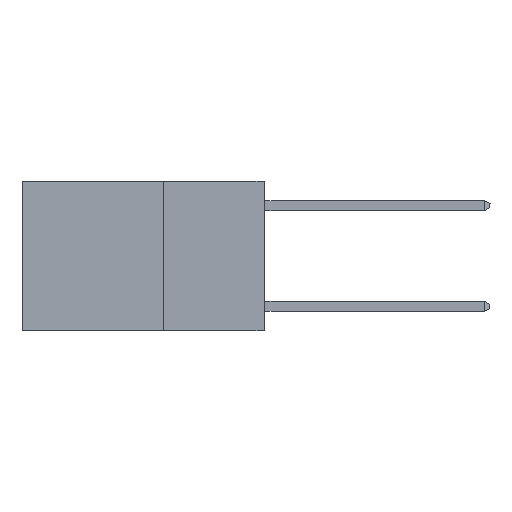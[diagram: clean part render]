
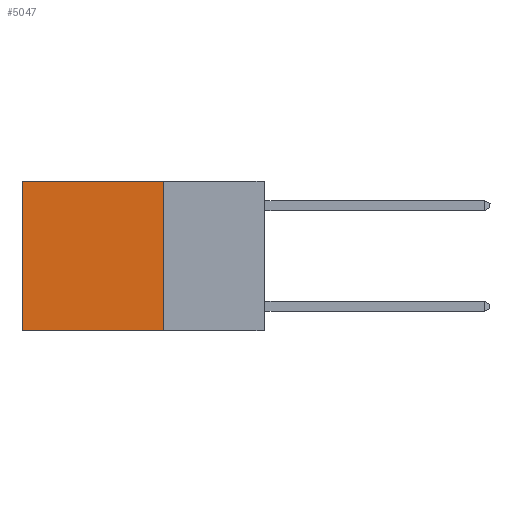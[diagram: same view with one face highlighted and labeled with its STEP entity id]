
A CAD part, left-side view. The second image highlights one B-rep face of the part: STEP entity #5047.
In plain terms, the highlighted planar face has unit normal (-1, 0, 0).
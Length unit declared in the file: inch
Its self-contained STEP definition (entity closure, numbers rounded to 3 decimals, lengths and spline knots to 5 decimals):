
#26 = DIRECTION ( 'NONE',  ( 0., 1., 0. ) ) ;
#517 = ORIENTED_EDGE ( 'NONE', *, *, #11591, .F. ) ;
#557 = ORIENTED_EDGE ( 'NONE', *, *, #10270, .T. ) ;
#686 = VECTOR ( 'NONE', #26, 39.37008 ) ;
#772 = ORIENTED_EDGE ( 'NONE', *, *, #4914, .F. ) ;
#889 = ORIENTED_EDGE ( 'NONE', *, *, #3228, .T. ) ;
#1190 = VERTEX_POINT ( 'NONE', #11742 ) ;
#1221 = VERTEX_POINT ( 'NONE', #10866 ) ;
#1731 = DIRECTION ( 'NONE',  ( 0., 0., -1. ) ) ;
#3228 = EDGE_CURVE ( 'NONE', #4956, #6445, #5543, .T. ) ;
#3230 = AXIS2_PLACEMENT_3D ( 'NONE', #3625, #7593, #1731 ) ;
#3414 = CARTESIAN_POINT ( 'NONE',  ( 0.2625, 0.25, 0. ) ) ;
#3625 = CARTESIAN_POINT ( 'NONE',  ( 0.2625, 0.25, 0. ) ) ;
#4360 = CARTESIAN_POINT ( 'NONE',  ( 0.2625, 0.25, 0. ) ) ;
#4914 = EDGE_CURVE ( 'NONE', #4956, #1221, #7674, .T. ) ;
#4956 = VERTEX_POINT ( 'NONE', #3414 ) ;
#5047 = ADVANCED_FACE ( 'NONE', ( #10923 ), #6607, .F. ) ;
#5053 = VECTOR ( 'NONE', #11059, 39.37008 ) ;
#5543 = LINE ( 'NONE', #4360, #686 ) ;
#5617 = VECTOR ( 'NONE', #12389, 39.37008 ) ;
#6211 = DIRECTION ( 'NONE',  ( 0., 0., -1. ) ) ;
#6445 = VERTEX_POINT ( 'NONE', #10178 ) ;
#6607 = PLANE ( 'NONE',  #3230 ) ;
#6816 = EDGE_LOOP ( 'NONE', ( #557, #517, #772, #889 ) ) ;
#7593 = DIRECTION ( 'NONE',  ( 1., 0., 0. ) ) ;
#7674 = LINE ( 'NONE', #9155, #5053 ) ;
#7915 = LINE ( 'NONE', #8662, #5617 ) ;
#8662 = CARTESIAN_POINT ( 'NONE',  ( 0.2625, 0.25, -0.37 ) ) ;
#9155 = CARTESIAN_POINT ( 'NONE',  ( 0.2625, 0.25, 0. ) ) ;
#9575 = LINE ( 'NONE', #11902, #11493 ) ;
#10178 = CARTESIAN_POINT ( 'NONE',  ( 0.2625, 0.6, 0. ) ) ;
#10270 = EDGE_CURVE ( 'NONE', #6445, #1190, #9575, .T. ) ;
#10866 = CARTESIAN_POINT ( 'NONE',  ( 0.2625, 0.25, -0.37 ) ) ;
#10923 = FACE_OUTER_BOUND ( 'NONE', #6816, .T. ) ;
#11059 = DIRECTION ( 'NONE',  ( 0., 0., -1. ) ) ;
#11493 = VECTOR ( 'NONE', #6211, 39.37008 ) ;
#11591 = EDGE_CURVE ( 'NONE', #1221, #1190, #7915, .T. ) ;
#11742 = CARTESIAN_POINT ( 'NONE',  ( 0.2625, 0.6, -0.37 ) ) ;
#11902 = CARTESIAN_POINT ( 'NONE',  ( 0.2625, 0.6, 0. ) ) ;
#12389 = DIRECTION ( 'NONE',  ( 0., 1., 0. ) ) ;
